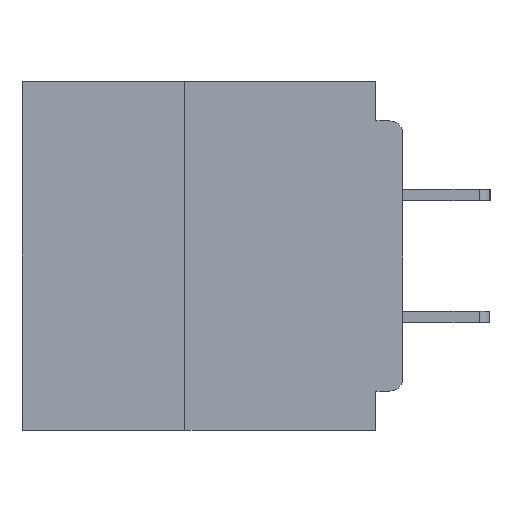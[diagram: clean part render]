
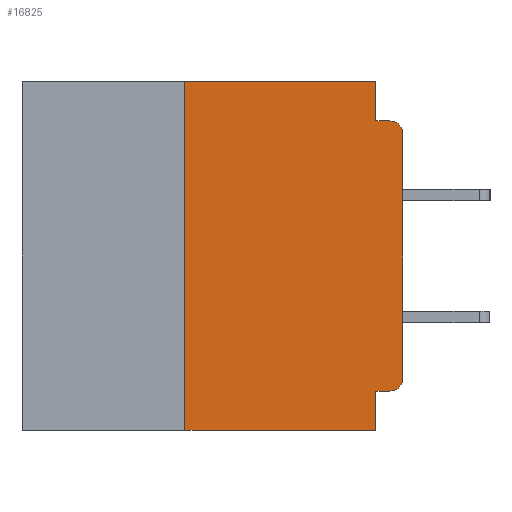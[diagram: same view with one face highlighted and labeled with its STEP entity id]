
A CAD part, left-side view. The second image highlights one B-rep face of the part: STEP entity #16825.
In plain terms, the highlighted planar face has unit normal (-1, 0, 0).
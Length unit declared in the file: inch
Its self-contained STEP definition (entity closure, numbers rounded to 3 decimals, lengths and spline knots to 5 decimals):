
#221 = EDGE_CURVE ( 'NONE', #5091, #32283, #22625, .T. ) ;
#255 = DIRECTION ( 'NONE',  ( 0., 0., 1. ) ) ;
#967 = LINE ( 'NONE', #16619, #18820 ) ;
#1842 = DIRECTION ( 'NONE',  ( 0., 0., -1. ) ) ;
#2005 = PLANE ( 'NONE',  #32288 ) ;
#2181 = EDGE_LOOP ( 'NONE', ( #39593, #13420, #4876, #27564, #11765, #31342, #37295, #31262, #5713, #13614 ) ) ;
#2548 = LINE ( 'NONE', #5389, #3036 ) ;
#3014 = VECTOR ( 'NONE', #1842, 39.37008 ) ;
#3036 = VECTOR ( 'NONE', #30229, 39.37008 ) ;
#3101 = CARTESIAN_POINT ( 'NONE',  ( 0., 0.031, -0.355 ) ) ;
#3639 = VECTOR ( 'NONE', #31230, 39.37008 ) ;
#3733 = CARTESIAN_POINT ( 'NONE',  ( 0., 0.031, -0.4 ) ) ;
#4876 = ORIENTED_EDGE ( 'NONE', *, *, #25621, .F. ) ;
#5091 = VERTEX_POINT ( 'NONE', #15688 ) ;
#5389 = CARTESIAN_POINT ( 'NONE',  ( 0., 0.437, 0. ) ) ;
#5628 = EDGE_CURVE ( 'NONE', #26714, #32283, #967, .T. ) ;
#5713 = ORIENTED_EDGE ( 'NONE', *, *, #16164, .F. ) ;
#6457 = CARTESIAN_POINT ( 'NONE',  ( 0., 0.015, -0.06 ) ) ;
#6866 = EDGE_CURVE ( 'NONE', #37856, #9729, #2548, .T. ) ;
#7389 = VECTOR ( 'NONE', #24128, 39.37008 ) ;
#7693 = VERTEX_POINT ( 'NONE', #34790 ) ;
#7790 = CARTESIAN_POINT ( 'NONE',  ( 0., 0.015, -0.045 ) ) ;
#9161 = DIRECTION ( 'NONE',  ( 0., 0., -1. ) ) ;
#9523 = VECTOR ( 'NONE', #44218, 39.37008 ) ;
#9729 = VERTEX_POINT ( 'NONE', #41880 ) ;
#9945 = CARTESIAN_POINT ( 'NONE',  ( 0., 0., -0.045 ) ) ;
#10037 = DIRECTION ( 'NONE',  ( 0., 0., -1. ) ) ;
#11765 = ORIENTED_EDGE ( 'NONE', *, *, #6866, .F. ) ;
#12272 = DIRECTION ( 'NONE',  ( -1., 0., 0. ) ) ;
#12522 = LINE ( 'NONE', #44308, #3014 ) ;
#12859 = CARTESIAN_POINT ( 'NONE',  ( 0., 0.437, -0.4 ) ) ;
#13261 = CARTESIAN_POINT ( 'NONE',  ( 0., 0., -0.34 ) ) ;
#13420 = ORIENTED_EDGE ( 'NONE', *, *, #24419, .T. ) ;
#13489 = DIRECTION ( 'NONE',  ( 0., 0., -1. ) ) ;
#13614 = ORIENTED_EDGE ( 'NONE', *, *, #29621, .T. ) ;
#15688 = CARTESIAN_POINT ( 'NONE',  ( 0., 0.25, -0.4 ) ) ;
#16164 = EDGE_CURVE ( 'NONE', #21736, #26714, #20155, .T. ) ;
#16619 = CARTESIAN_POINT ( 'NONE',  ( 0., 0.031, -0.4 ) ) ;
#16810 = EDGE_CURVE ( 'NONE', #9729, #29162, #12522, .T. ) ;
#16825 = ADVANCED_FACE ( 'NONE', ( #30257 ), #2005, .F. ) ;
#17019 = CARTESIAN_POINT ( 'NONE',  ( 0., 0.031, -0.045 ) ) ;
#17703 = AXIS2_PLACEMENT_3D ( 'NONE', #33486, #12272, #37050 ) ;
#17985 = DIRECTION ( 'NONE',  ( 0., -1., 0. ) ) ;
#18820 = VECTOR ( 'NONE', #13489, 39.37008 ) ;
#18955 = LINE ( 'NONE', #32221, #35513 ) ;
#20026 = VERTEX_POINT ( 'NONE', #7790 ) ;
#20155 = LINE ( 'NONE', #23103, #9523 ) ;
#20364 = LINE ( 'NONE', #9945, #3639 ) ;
#21736 = VERTEX_POINT ( 'NONE', #34206 ) ;
#22625 = LINE ( 'NONE', #12859, #40286 ) ;
#23103 = CARTESIAN_POINT ( 'NONE',  ( 0., 0., -0.355 ) ) ;
#24128 = DIRECTION ( 'NONE',  ( 0., 0., 1. ) ) ;
#24419 = EDGE_CURVE ( 'NONE', #7693, #20026, #42019, .T. ) ;
#25621 = EDGE_CURVE ( 'NONE', #29162, #20026, #20364, .T. ) ;
#26714 = VERTEX_POINT ( 'NONE', #3101 ) ;
#27564 = ORIENTED_EDGE ( 'NONE', *, *, #16810, .F. ) ;
#27685 = CARTESIAN_POINT ( 'NONE',  ( 0., 0.25, -0.4 ) ) ;
#28532 = LINE ( 'NONE', #27685, #7389 ) ;
#29110 = CIRCLE ( 'NONE', #17703, 0.015 ) ;
#29162 = VERTEX_POINT ( 'NONE', #17019 ) ;
#29621 = EDGE_CURVE ( 'NONE', #21736, #31169, #29110, .T. ) ;
#30229 = DIRECTION ( 'NONE',  ( 0., -1., 0. ) ) ;
#30257 = FACE_OUTER_BOUND ( 'NONE', #2181, .T. ) ;
#30443 = DIRECTION ( 'NONE',  ( 1., 0., 0. ) ) ;
#31169 = VERTEX_POINT ( 'NONE', #13261 ) ;
#31230 = DIRECTION ( 'NONE',  ( 0., -1., 0. ) ) ;
#31262 = ORIENTED_EDGE ( 'NONE', *, *, #5628, .F. ) ;
#31320 = DIRECTION ( 'NONE',  ( -1., 0., 0. ) ) ;
#31342 = ORIENTED_EDGE ( 'NONE', *, *, #45510, .F. ) ;
#32221 = CARTESIAN_POINT ( 'NONE',  ( 0., 0., 0. ) ) ;
#32283 = VERTEX_POINT ( 'NONE', #3733 ) ;
#32288 = AXIS2_PLACEMENT_3D ( 'NONE', #44466, #30443, #9161 ) ;
#33486 = CARTESIAN_POINT ( 'NONE',  ( 0., 0.015, -0.34 ) ) ;
#34206 = CARTESIAN_POINT ( 'NONE',  ( 0., 0.015, -0.355 ) ) ;
#34790 = CARTESIAN_POINT ( 'NONE',  ( 0., 0., -0.06 ) ) ;
#35513 = VECTOR ( 'NONE', #255, 39.37008 ) ;
#37050 = DIRECTION ( 'NONE',  ( 0., 0., -1. ) ) ;
#37295 = ORIENTED_EDGE ( 'NONE', *, *, #221, .T. ) ;
#37496 = CARTESIAN_POINT ( 'NONE',  ( 0., 0.25, 0. ) ) ;
#37856 = VERTEX_POINT ( 'NONE', #37496 ) ;
#38307 = AXIS2_PLACEMENT_3D ( 'NONE', #6457, #31320, #10037 ) ;
#39593 = ORIENTED_EDGE ( 'NONE', *, *, #41776, .T. ) ;
#40286 = VECTOR ( 'NONE', #17985, 39.37008 ) ;
#41776 = EDGE_CURVE ( 'NONE', #31169, #7693, #18955, .T. ) ;
#41880 = CARTESIAN_POINT ( 'NONE',  ( 0., 0.031, 0. ) ) ;
#42019 = CIRCLE ( 'NONE', #38307, 0.015 ) ;
#44218 = DIRECTION ( 'NONE',  ( 0., 1., 0. ) ) ;
#44308 = CARTESIAN_POINT ( 'NONE',  ( 0., 0.031, 0. ) ) ;
#44466 = CARTESIAN_POINT ( 'NONE',  ( 0., 0.437, 0. ) ) ;
#45510 = EDGE_CURVE ( 'NONE', #5091, #37856, #28532, .T. ) ;
